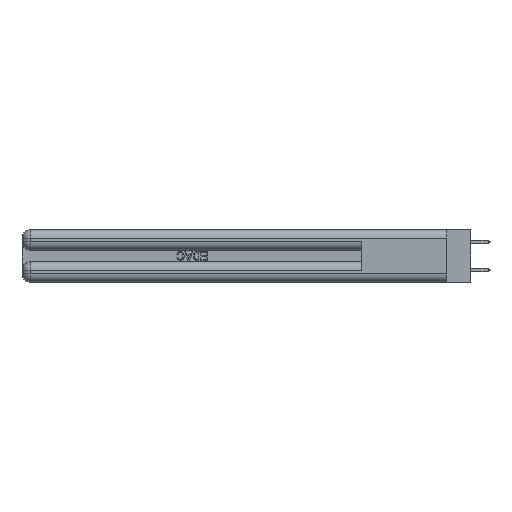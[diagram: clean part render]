
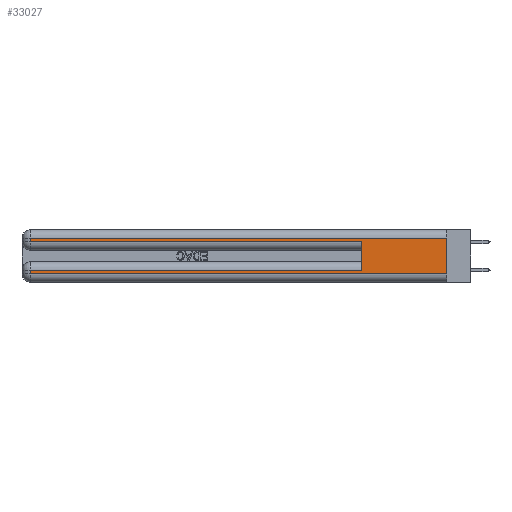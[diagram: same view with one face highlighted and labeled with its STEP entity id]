
A CAD part, left-side view. The second image highlights one B-rep face of the part: STEP entity #33027.
In plain terms, the highlighted planar face has unit normal (-1, 0, 0).
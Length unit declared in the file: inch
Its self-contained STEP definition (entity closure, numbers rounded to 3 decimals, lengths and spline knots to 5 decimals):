
#37 = CARTESIAN_POINT ( 'NONE',  ( 0., 2.94, 0.285 ) ) ;
#304 = ORIENTED_EDGE ( 'NONE', *, *, #29057, .T. ) ;
#307 = ORIENTED_EDGE ( 'NONE', *, *, #40486, .F. ) ;
#702 = VERTEX_POINT ( 'NONE', #31240 ) ;
#731 = LINE ( 'NONE', #14671, #11598 ) ;
#846 = DIRECTION ( 'NONE',  ( 0., 0., -1. ) ) ;
#968 = CARTESIAN_POINT ( 'NONE',  ( 0., 2.94, 0.31 ) ) ;
#2785 = VECTOR ( 'NONE', #22720, 39.37008 ) ;
#2911 = DIRECTION ( 'NONE',  ( 0., 0., -1. ) ) ;
#3117 = FACE_OUTER_BOUND ( 'NONE', #10600, .T. ) ;
#3363 = CARTESIAN_POINT ( 'NONE',  ( 0., 2.94, 0.085 ) ) ;
#3519 = CARTESIAN_POINT ( 'NONE',  ( 0., 0., 0.37 ) ) ;
#5873 = ORIENTED_EDGE ( 'NONE', *, *, #23751, .F. ) ;
#6315 = ORIENTED_EDGE ( 'NONE', *, *, #10368, .T. ) ;
#6680 = LINE ( 'NONE', #31119, #35914 ) ;
#6787 = EDGE_CURVE ( 'NONE', #11943, #702, #31664, .T. ) ;
#6962 = VECTOR ( 'NONE', #25561, 39.37008 ) ;
#8041 = LINE ( 'NONE', #26752, #31334 ) ;
#8270 = DIRECTION ( 'NONE',  ( 0., -1., 0. ) ) ;
#8873 = VERTEX_POINT ( 'NONE', #968 ) ;
#9836 = DIRECTION ( 'NONE',  ( 0., 0., -1. ) ) ;
#10368 = EDGE_CURVE ( 'NONE', #29047, #14875, #731, .T. ) ;
#10600 = EDGE_LOOP ( 'NONE', ( #307, #25282, #304, #6315, #5873, #23137, #36787, #15034 ) ) ;
#11598 = VECTOR ( 'NONE', #8270, 39.37008 ) ;
#11943 = VERTEX_POINT ( 'NONE', #3363 ) ;
#12045 = VECTOR ( 'NONE', #20811, 39.37008 ) ;
#14198 = CARTESIAN_POINT ( 'NONE',  ( 0., 0., 0.06 ) ) ;
#14671 = CARTESIAN_POINT ( 'NONE',  ( 0., 0., 0.285 ) ) ;
#14875 = VERTEX_POINT ( 'NONE', #28723 ) ;
#15034 = ORIENTED_EDGE ( 'NONE', *, *, #25905, .T. ) ;
#15415 = LINE ( 'NONE', #22449, #6962 ) ;
#15619 = CARTESIAN_POINT ( 'NONE',  ( 0., 0., 0.31 ) ) ;
#17781 = CARTESIAN_POINT ( 'NONE',  ( 0., 0.6, 0.145 ) ) ;
#19835 = CARTESIAN_POINT ( 'NONE',  ( 0., 0., 0.37 ) ) ;
#20055 = EDGE_CURVE ( 'NONE', #39754, #11943, #8041, .T. ) ;
#20811 = DIRECTION ( 'NONE',  ( 0., 0., 1. ) ) ;
#21051 = LINE ( 'NONE', #19835, #26419 ) ;
#22134 = AXIS2_PLACEMENT_3D ( 'NONE', #3519, #25602, #9836 ) ;
#22449 = CARTESIAN_POINT ( 'NONE',  ( 0., 0., 0.06 ) ) ;
#22720 = DIRECTION ( 'NONE',  ( 0., 0., -1. ) ) ;
#22798 = CARTESIAN_POINT ( 'NONE',  ( 0., 0.6, 0.085 ) ) ;
#22815 = DIRECTION ( 'NONE',  ( 0., 1., 0. ) ) ;
#23137 = ORIENTED_EDGE ( 'NONE', *, *, #20055, .T. ) ;
#23751 = EDGE_CURVE ( 'NONE', #39754, #14875, #30342, .T. ) ;
#23752 = DIRECTION ( 'NONE',  ( 0., 1., 0. ) ) ;
#25282 = ORIENTED_EDGE ( 'NONE', *, *, #27349, .T. ) ;
#25561 = DIRECTION ( 'NONE',  ( 0., -1., 0. ) ) ;
#25602 = DIRECTION ( 'NONE',  ( 1., 0., 0. ) ) ;
#25905 = EDGE_CURVE ( 'NONE', #702, #27586, #15415, .T. ) ;
#26419 = VECTOR ( 'NONE', #846, 39.37008 ) ;
#26752 = CARTESIAN_POINT ( 'NONE',  ( 0., 0., 0.085 ) ) ;
#27349 = EDGE_CURVE ( 'NONE', #37737, #8873, #30601, .T. ) ;
#27586 = VERTEX_POINT ( 'NONE', #14198 ) ;
#28723 = CARTESIAN_POINT ( 'NONE',  ( 0., 0.6, 0.285 ) ) ;
#29047 = VERTEX_POINT ( 'NONE', #37 ) ;
#29057 = EDGE_CURVE ( 'NONE', #8873, #29047, #6680, .T. ) ;
#30342 = LINE ( 'NONE', #17781, #12045 ) ;
#30601 = LINE ( 'NONE', #15619, #40556 ) ;
#31119 = CARTESIAN_POINT ( 'NONE',  ( 0., 2.94, 0.37 ) ) ;
#31240 = CARTESIAN_POINT ( 'NONE',  ( 0., 2.94, 0.06 ) ) ;
#31334 = VECTOR ( 'NONE', #23752, 39.37008 ) ;
#31664 = LINE ( 'NONE', #40316, #2785 ) ;
#33027 = ADVANCED_FACE ( 'NONE', ( #3117 ), #38330, .F. ) ;
#34851 = CARTESIAN_POINT ( 'NONE',  ( 0., 0., 0.31 ) ) ;
#35914 = VECTOR ( 'NONE', #2911, 39.37008 ) ;
#36787 = ORIENTED_EDGE ( 'NONE', *, *, #6787, .T. ) ;
#37737 = VERTEX_POINT ( 'NONE', #34851 ) ;
#38330 = PLANE ( 'NONE',  #22134 ) ;
#39754 = VERTEX_POINT ( 'NONE', #22798 ) ;
#40316 = CARTESIAN_POINT ( 'NONE',  ( 0., 2.94, 0.37 ) ) ;
#40486 = EDGE_CURVE ( 'NONE', #37737, #27586, #21051, .T. ) ;
#40556 = VECTOR ( 'NONE', #22815, 39.37008 ) ;
